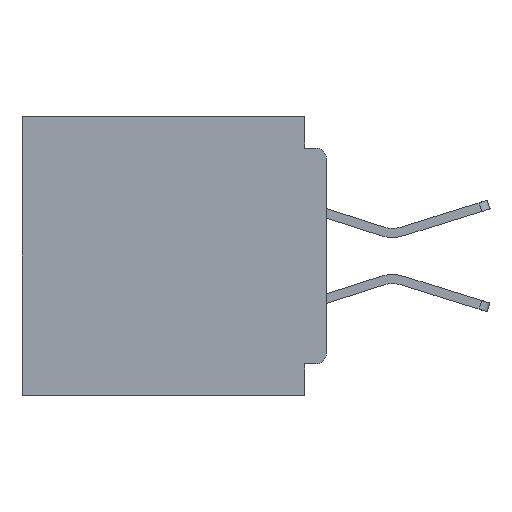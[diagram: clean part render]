
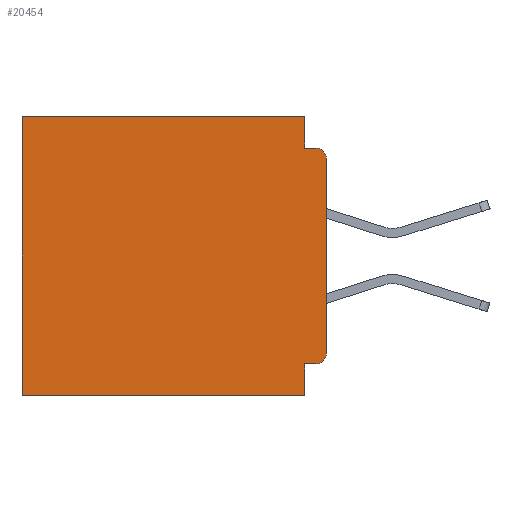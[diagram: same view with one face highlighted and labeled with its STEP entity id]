
A CAD part, left-side view. The second image highlights one B-rep face of the part: STEP entity #20454.
In plain terms, the highlighted planar face has unit normal (-1, 0, 0).
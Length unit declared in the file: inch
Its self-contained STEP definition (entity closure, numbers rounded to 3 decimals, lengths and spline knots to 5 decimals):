
#84 = LINE ( 'NONE', #53156, #43130 ) ;
#1587 = VERTEX_POINT ( 'NONE', #14683 ) ;
#2490 = VECTOR ( 'NONE', #45060, 39.37008 ) ;
#2839 = DIRECTION ( 'NONE',  ( 0., 0., -1. ) ) ;
#3305 = VECTOR ( 'NONE', #45915, 39.37008 ) ;
#3756 = LINE ( 'NONE', #31768, #24620 ) ;
#4564 = DIRECTION ( 'NONE',  ( -1., 0., 0. ) ) ;
#4650 = PLANE ( 'NONE',  #21728 ) ;
#5318 = DIRECTION ( 'NONE',  ( 0., 1., 0. ) ) ;
#8076 = CARTESIAN_POINT ( 'NONE',  ( 0.3, 0.015, -0.355 ) ) ;
#8601 = EDGE_CURVE ( 'NONE', #11420, #42443, #35816, .T. ) ;
#8649 = AXIS2_PLACEMENT_3D ( 'NONE', #52712, #27814, #2839 ) ;
#8779 = VERTEX_POINT ( 'NONE', #50292 ) ;
#8871 = DIRECTION ( 'NONE',  ( 1., 0., 0. ) ) ;
#10094 = EDGE_LOOP ( 'NONE', ( #17434, #50088, #27251, #42765, #14422, #17332, #28943, #17979, #21718, #31408 ) ) ;
#10541 = EDGE_CURVE ( 'NONE', #8779, #26164, #14787, .T. ) ;
#11420 = VERTEX_POINT ( 'NONE', #13564 ) ;
#12814 = CIRCLE ( 'NONE', #8649, 0.015 ) ;
#12986 = CARTESIAN_POINT ( 'NONE',  ( 0.3, 0.031, -0.4 ) ) ;
#13504 = EDGE_CURVE ( 'NONE', #40546, #22139, #84, .T. ) ;
#13564 = CARTESIAN_POINT ( 'NONE',  ( 0.3, 0.031, -0.045 ) ) ;
#14048 = CARTESIAN_POINT ( 'NONE',  ( 0.3, 0., -0.4 ) ) ;
#14422 = ORIENTED_EDGE ( 'NONE', *, *, #39323, .T. ) ;
#14630 = EDGE_CURVE ( 'NONE', #26499, #11420, #3756, .T. ) ;
#14683 = CARTESIAN_POINT ( 'NONE',  ( 0.3, 0., -0.06 ) ) ;
#14787 = LINE ( 'NONE', #32390, #46666 ) ;
#14844 = VECTOR ( 'NONE', #21684, 39.37008 ) ;
#15998 = EDGE_CURVE ( 'NONE', #24772, #29953, #12814, .T. ) ;
#16357 = VECTOR ( 'NONE', #26371, 39.37008 ) ;
#17332 = ORIENTED_EDGE ( 'NONE', *, *, #13504, .T. ) ;
#17434 = ORIENTED_EDGE ( 'NONE', *, *, #50560, .F. ) ;
#17979 = ORIENTED_EDGE ( 'NONE', *, *, #10541, .F. ) ;
#18709 = CARTESIAN_POINT ( 'NONE',  ( 0.3, 0., -0.34 ) ) ;
#19416 = EDGE_CURVE ( 'NONE', #26164, #22139, #39834, .T. ) ;
#20454 = ADVANCED_FACE ( 'NONE', ( #45418 ), #4650, .F. ) ;
#21206 = CARTESIAN_POINT ( 'NONE',  ( 0.3, 0.437, 0. ) ) ;
#21684 = DIRECTION ( 'NONE',  ( 0., 1., 0. ) ) ;
#21718 = ORIENTED_EDGE ( 'NONE', *, *, #40688, .F. ) ;
#21728 = AXIS2_PLACEMENT_3D ( 'NONE', #41870, #8871, #38031 ) ;
#22139 = VERTEX_POINT ( 'NONE', #40639 ) ;
#23509 = CARTESIAN_POINT ( 'NONE',  ( 0.3, 0.031, 0. ) ) ;
#24280 = DIRECTION ( 'NONE',  ( 0., 0., -1. ) ) ;
#24620 = VECTOR ( 'NONE', #36020, 39.37008 ) ;
#24772 = VERTEX_POINT ( 'NONE', #8076 ) ;
#25795 = CIRCLE ( 'NONE', #46463, 0.015 ) ;
#25878 = LINE ( 'NONE', #38109, #14844 ) ;
#26164 = VERTEX_POINT ( 'NONE', #12986 ) ;
#26371 = DIRECTION ( 'NONE',  ( 0., 1., 0. ) ) ;
#26499 = VERTEX_POINT ( 'NONE', #23509 ) ;
#26755 = LINE ( 'NONE', #29319, #3305 ) ;
#27251 = ORIENTED_EDGE ( 'NONE', *, *, #8601, .F. ) ;
#27814 = DIRECTION ( 'NONE',  ( -1., 0., 0. ) ) ;
#28943 = ORIENTED_EDGE ( 'NONE', *, *, #19416, .F. ) ;
#29319 = CARTESIAN_POINT ( 'NONE',  ( 0.3, 0., -0.4 ) ) ;
#29454 = CARTESIAN_POINT ( 'NONE',  ( 0.3, 0.015, -0.06 ) ) ;
#29953 = VERTEX_POINT ( 'NONE', #18709 ) ;
#31408 = ORIENTED_EDGE ( 'NONE', *, *, #15998, .T. ) ;
#31768 = CARTESIAN_POINT ( 'NONE',  ( 0.3, 0.031, 0. ) ) ;
#32390 = CARTESIAN_POINT ( 'NONE',  ( 0.3, 0.031, -0.4 ) ) ;
#33728 = DIRECTION ( 'NONE',  ( 0., 0., -1. ) ) ;
#35816 = LINE ( 'NONE', #40924, #2490 ) ;
#36020 = DIRECTION ( 'NONE',  ( 0., 0., -1. ) ) ;
#36352 = EDGE_CURVE ( 'NONE', #1587, #42443, #25795, .T. ) ;
#38031 = DIRECTION ( 'NONE',  ( 0., 0., -1. ) ) ;
#38109 = CARTESIAN_POINT ( 'NONE',  ( 0.3, 0., 0. ) ) ;
#39323 = EDGE_CURVE ( 'NONE', #26499, #40546, #25878, .T. ) ;
#39834 = LINE ( 'NONE', #14048, #16357 ) ;
#40546 = VERTEX_POINT ( 'NONE', #21206 ) ;
#40639 = CARTESIAN_POINT ( 'NONE',  ( 0.3, 0.437, -0.4 ) ) ;
#40688 = EDGE_CURVE ( 'NONE', #24772, #8779, #46021, .T. ) ;
#40924 = CARTESIAN_POINT ( 'NONE',  ( 0.3, 0., -0.045 ) ) ;
#41870 = CARTESIAN_POINT ( 'NONE',  ( 0.3, 0., -0.4 ) ) ;
#42443 = VERTEX_POINT ( 'NONE', #48151 ) ;
#42698 = CARTESIAN_POINT ( 'NONE',  ( 0.3, 0., -0.355 ) ) ;
#42765 = ORIENTED_EDGE ( 'NONE', *, *, #14630, .F. ) ;
#43130 = VECTOR ( 'NONE', #24280, 39.37008 ) ;
#44733 = VECTOR ( 'NONE', #5318, 39.37008 ) ;
#44984 = DIRECTION ( 'NONE',  ( 0., 0., -1. ) ) ;
#45060 = DIRECTION ( 'NONE',  ( 0., -1., 0. ) ) ;
#45418 = FACE_OUTER_BOUND ( 'NONE', #10094, .T. ) ;
#45915 = DIRECTION ( 'NONE',  ( 0., 0., -1. ) ) ;
#46021 = LINE ( 'NONE', #42698, #44733 ) ;
#46463 = AXIS2_PLACEMENT_3D ( 'NONE', #29454, #4564, #33728 ) ;
#46666 = VECTOR ( 'NONE', #44984, 39.37008 ) ;
#48151 = CARTESIAN_POINT ( 'NONE',  ( 0.3, 0.015, -0.045 ) ) ;
#50088 = ORIENTED_EDGE ( 'NONE', *, *, #36352, .T. ) ;
#50292 = CARTESIAN_POINT ( 'NONE',  ( 0.3, 0.031, -0.355 ) ) ;
#50560 = EDGE_CURVE ( 'NONE', #1587, #29953, #26755, .T. ) ;
#52712 = CARTESIAN_POINT ( 'NONE',  ( 0.3, 0.015, -0.34 ) ) ;
#53156 = CARTESIAN_POINT ( 'NONE',  ( 0.3, 0.437, -0.4 ) ) ;
